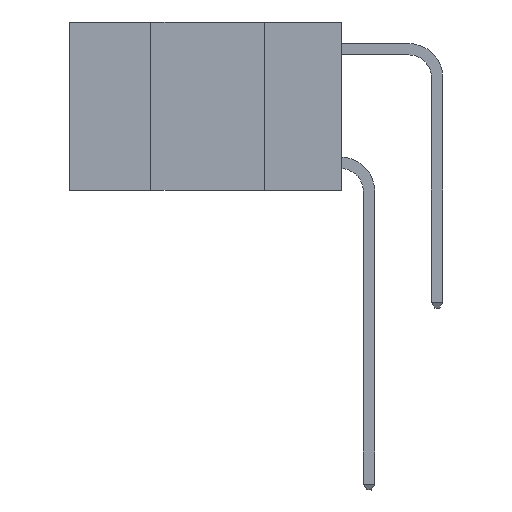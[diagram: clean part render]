
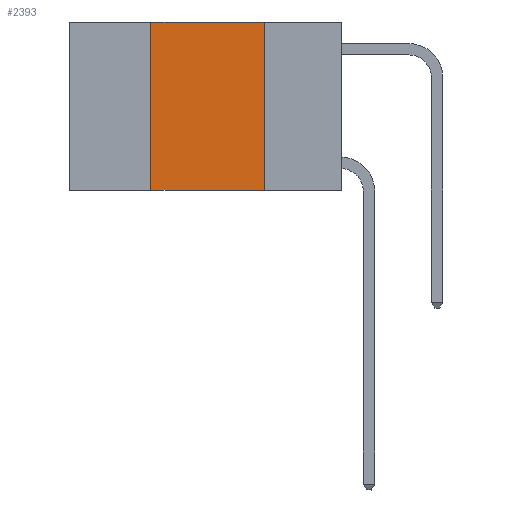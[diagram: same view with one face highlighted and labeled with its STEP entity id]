
A CAD part, left-side view. The second image highlights one B-rep face of the part: STEP entity #2393.
In plain terms, the highlighted planar face has unit normal (-1, 0, 0).
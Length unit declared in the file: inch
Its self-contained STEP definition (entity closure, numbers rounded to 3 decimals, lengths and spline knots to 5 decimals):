
#217 = VECTOR ( 'NONE', #1890, 39.37008 ) ;
#479 = VERTEX_POINT ( 'NONE', #8196 ) ;
#804 = VECTOR ( 'NONE', #2172, 39.37008 ) ;
#968 = VERTEX_POINT ( 'NONE', #1140 ) ;
#1001 = LINE ( 'NONE', #2263, #804 ) ;
#1140 = CARTESIAN_POINT ( 'NONE',  ( 0., 0.17, -0.37 ) ) ;
#1279 = DIRECTION ( 'NONE',  ( 0., 0., -1. ) ) ;
#1290 = CARTESIAN_POINT ( 'NONE',  ( 0., 0.17, 0. ) ) ;
#1588 = LINE ( 'NONE', #1870, #217 ) ;
#1870 = CARTESIAN_POINT ( 'NONE',  ( 0., 0.42, 0. ) ) ;
#1890 = DIRECTION ( 'NONE',  ( 0., 0., 1. ) ) ;
#1915 = ORIENTED_EDGE ( 'NONE', *, *, #8607, .T. ) ;
#2072 = CARTESIAN_POINT ( 'NONE',  ( 0., 0.42, -0.37 ) ) ;
#2172 = DIRECTION ( 'NONE',  ( 0., -1., 0. ) ) ;
#2263 = CARTESIAN_POINT ( 'NONE',  ( 0., 0.6, -0.37 ) ) ;
#2393 = ADVANCED_FACE ( 'NONE', ( #4439 ), #7919, .F. ) ;
#3558 = ORIENTED_EDGE ( 'NONE', *, *, #8732, .F. ) ;
#3767 = VERTEX_POINT ( 'NONE', #2072 ) ;
#4417 = CARTESIAN_POINT ( 'NONE',  ( 0., 0.42, 0. ) ) ;
#4428 = VECTOR ( 'NONE', #7278, 39.37008 ) ;
#4433 = LINE ( 'NONE', #7354, #4428 ) ;
#4439 = FACE_OUTER_BOUND ( 'NONE', #5985, .T. ) ;
#4483 = AXIS2_PLACEMENT_3D ( 'NONE', #6991, #6424, #6118 ) ;
#4608 = EDGE_CURVE ( 'NONE', #4980, #479, #4433, .T. ) ;
#4646 = LINE ( 'NONE', #1290, #10035 ) ;
#4980 = VERTEX_POINT ( 'NONE', #4417 ) ;
#5985 = EDGE_LOOP ( 'NONE', ( #8528, #9730, #3558, #1915 ) ) ;
#6118 = DIRECTION ( 'NONE',  ( 0., 0., -1. ) ) ;
#6424 = DIRECTION ( 'NONE',  ( 1., 0., 0. ) ) ;
#6991 = CARTESIAN_POINT ( 'NONE',  ( 0., 0.6, 0. ) ) ;
#7278 = DIRECTION ( 'NONE',  ( 0., -1., 0. ) ) ;
#7354 = CARTESIAN_POINT ( 'NONE',  ( 0., 0.6, 0. ) ) ;
#7919 = PLANE ( 'NONE',  #4483 ) ;
#8196 = CARTESIAN_POINT ( 'NONE',  ( 0., 0.17, 0. ) ) ;
#8528 = ORIENTED_EDGE ( 'NONE', *, *, #8840, .F. ) ;
#8607 = EDGE_CURVE ( 'NONE', #3767, #968, #1001, .T. ) ;
#8732 = EDGE_CURVE ( 'NONE', #3767, #4980, #1588, .T. ) ;
#8840 = EDGE_CURVE ( 'NONE', #479, #968, #4646, .T. ) ;
#9730 = ORIENTED_EDGE ( 'NONE', *, *, #4608, .F. ) ;
#10035 = VECTOR ( 'NONE', #1279, 39.37008 ) ;
